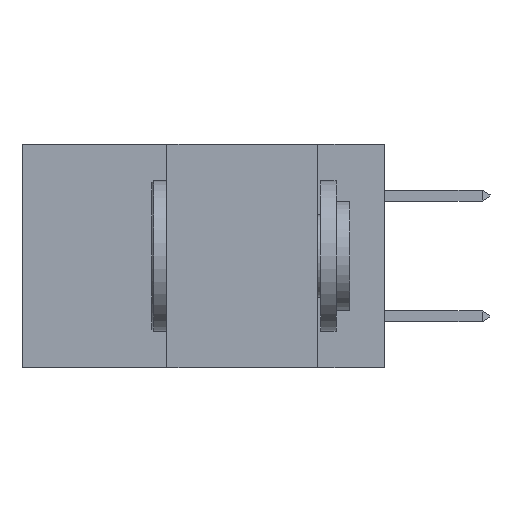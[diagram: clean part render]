
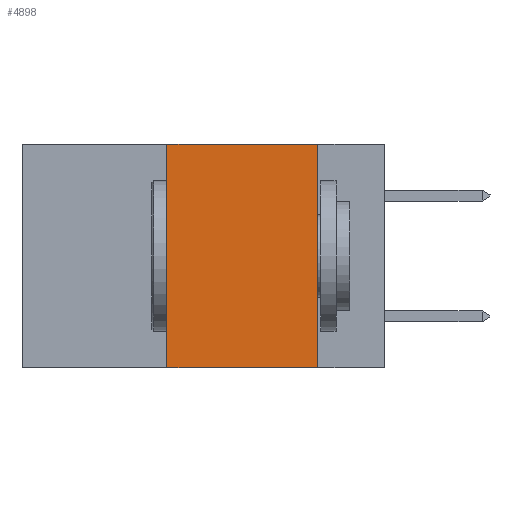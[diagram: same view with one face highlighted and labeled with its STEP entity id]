
A CAD part, left-side view. The second image highlights one B-rep face of the part: STEP entity #4898.
In plain terms, the highlighted planar face has unit normal (-1, 0, 0).
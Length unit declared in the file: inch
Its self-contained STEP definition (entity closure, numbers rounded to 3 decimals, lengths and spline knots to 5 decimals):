
#51 = CARTESIAN_POINT ( 'NONE',  ( 0., 0.11, 0. ) ) ;
#126 = DIRECTION ( 'NONE',  ( 0., -1., 0. ) ) ;
#327 = VERTEX_POINT ( 'NONE', #11538 ) ;
#743 = PLANE ( 'NONE',  #7198 ) ;
#1286 = VECTOR ( 'NONE', #126, 39.37008 ) ;
#1738 = CARTESIAN_POINT ( 'NONE',  ( 0., 0.6, -0.37 ) ) ;
#4898 = ADVANCED_FACE ( 'NONE', ( #19969 ), #743, .F. ) ;
#7198 = AXIS2_PLACEMENT_3D ( 'NONE', #19220, #24453, #8701 ) ;
#8701 = DIRECTION ( 'NONE',  ( 0., 0., -1. ) ) ;
#9520 = VECTOR ( 'NONE', #22799, 39.37008 ) ;
#10486 = ORIENTED_EDGE ( 'NONE', *, *, #27865, .F. ) ;
#10935 = EDGE_CURVE ( 'NONE', #11888, #14981, #23509, .T. ) ;
#11538 = CARTESIAN_POINT ( 'NONE',  ( 0., 0.11, 0. ) ) ;
#11880 = EDGE_CURVE ( 'NONE', #17239, #327, #21496, .T. ) ;
#11888 = VERTEX_POINT ( 'NONE', #18603 ) ;
#13326 = DIRECTION ( 'NONE',  ( 0., 0., -1. ) ) ;
#14981 = VERTEX_POINT ( 'NONE', #23985 ) ;
#17239 = VERTEX_POINT ( 'NONE', #24562 ) ;
#17620 = VECTOR ( 'NONE', #20297, 39.37008 ) ;
#18342 = ORIENTED_EDGE ( 'NONE', *, *, #10935, .T. ) ;
#18447 = LINE ( 'NONE', #33180, #17620 ) ;
#18603 = CARTESIAN_POINT ( 'NONE',  ( 0., 0.36, -0.37 ) ) ;
#19220 = CARTESIAN_POINT ( 'NONE',  ( 0., 0.6, 0. ) ) ;
#19969 = FACE_OUTER_BOUND ( 'NONE', #32744, .T. ) ;
#20297 = DIRECTION ( 'NONE',  ( 0., 0., 1. ) ) ;
#20413 = ORIENTED_EDGE ( 'NONE', *, *, #30350, .F. ) ;
#21496 = LINE ( 'NONE', #28966, #1286 ) ;
#22799 = DIRECTION ( 'NONE',  ( 0., -1., 0. ) ) ;
#22841 = VECTOR ( 'NONE', #13326, 39.37008 ) ;
#23509 = LINE ( 'NONE', #1738, #9520 ) ;
#23985 = CARTESIAN_POINT ( 'NONE',  ( 0., 0.11, -0.37 ) ) ;
#24453 = DIRECTION ( 'NONE',  ( 1., 0., 0. ) ) ;
#24470 = LINE ( 'NONE', #51, #22841 ) ;
#24562 = CARTESIAN_POINT ( 'NONE',  ( 0., 0.36, 0. ) ) ;
#27326 = ORIENTED_EDGE ( 'NONE', *, *, #11880, .F. ) ;
#27865 = EDGE_CURVE ( 'NONE', #11888, #17239, #18447, .T. ) ;
#28966 = CARTESIAN_POINT ( 'NONE',  ( 0., 0.6, 0. ) ) ;
#30350 = EDGE_CURVE ( 'NONE', #327, #14981, #24470, .T. ) ;
#32744 = EDGE_LOOP ( 'NONE', ( #20413, #27326, #10486, #18342 ) ) ;
#33180 = CARTESIAN_POINT ( 'NONE',  ( 0., 0.36, 0. ) ) ;
